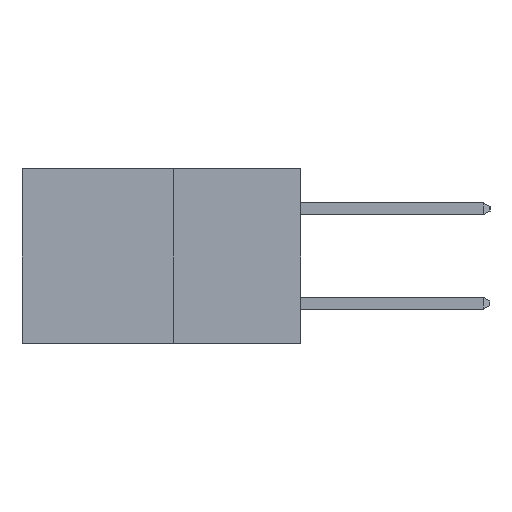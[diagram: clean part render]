
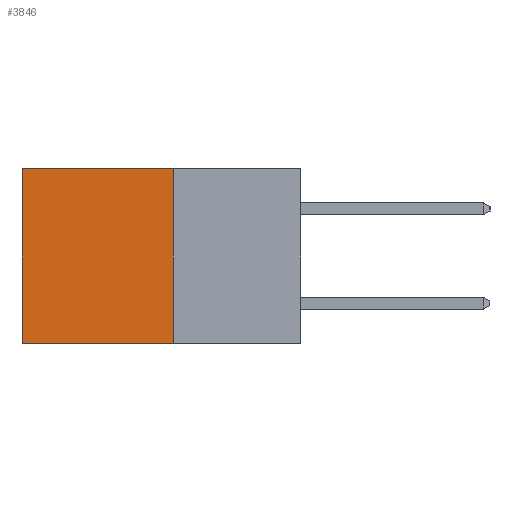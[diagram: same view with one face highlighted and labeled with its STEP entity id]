
A CAD part, left-side view. The second image highlights one B-rep face of the part: STEP entity #3846.
In plain terms, the highlighted planar face has unit normal (-1, 0, 0).
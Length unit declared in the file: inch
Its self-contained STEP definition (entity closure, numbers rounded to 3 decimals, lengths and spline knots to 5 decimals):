
#1355 = CARTESIAN_POINT ( 'NONE',  ( 0.277, 0.27, -0.37 ) ) ;
#2177 = LINE ( 'NONE', #3316, #24294 ) ;
#2244 = CARTESIAN_POINT ( 'NONE',  ( 0.277, 0.59, -0.37 ) ) ;
#3168 = EDGE_CURVE ( 'NONE', #17426, #20109, #24684, .T. ) ;
#3181 = DIRECTION ( 'NONE',  ( 0., 0., -1. ) ) ;
#3316 = CARTESIAN_POINT ( 'NONE',  ( 0.277, 0.59, -0.37 ) ) ;
#3846 = ADVANCED_FACE ( 'NONE', ( #8074 ), #18372, .F. ) ;
#5406 = ORIENTED_EDGE ( 'NONE', *, *, #13459, .F. ) ;
#6293 = EDGE_CURVE ( 'NONE', #20109, #27908, #2177, .T. ) ;
#6651 = EDGE_CURVE ( 'NONE', #17426, #11152, #9471, .T. ) ;
#7779 = VECTOR ( 'NONE', #15711, 39.37008 ) ;
#8074 = FACE_OUTER_BOUND ( 'NONE', #26539, .T. ) ;
#9471 = LINE ( 'NONE', #25321, #15317 ) ;
#11152 = VERTEX_POINT ( 'NONE', #25578 ) ;
#11865 = ORIENTED_EDGE ( 'NONE', *, *, #6651, .F. ) ;
#12144 = DIRECTION ( 'NONE',  ( 0., 0., -1. ) ) ;
#12700 = CARTESIAN_POINT ( 'NONE',  ( 0.277, 0.27, 0. ) ) ;
#12713 = ORIENTED_EDGE ( 'NONE', *, *, #3168, .T. ) ;
#12780 = CARTESIAN_POINT ( 'NONE',  ( 0.277, 0.59, 0. ) ) ;
#13048 = VECTOR ( 'NONE', #19036, 39.37008 ) ;
#13459 = EDGE_CURVE ( 'NONE', #11152, #27908, #19574, .T. ) ;
#14064 = ORIENTED_EDGE ( 'NONE', *, *, #6293, .T. ) ;
#15174 = AXIS2_PLACEMENT_3D ( 'NONE', #20018, #18273, #18241 ) ;
#15317 = VECTOR ( 'NONE', #12144, 39.37008 ) ;
#15711 = DIRECTION ( 'NONE',  ( 0., 1., 0. ) ) ;
#15801 = CARTESIAN_POINT ( 'NONE',  ( 0.277, 0.27, 0. ) ) ;
#17426 = VERTEX_POINT ( 'NONE', #12700 ) ;
#18241 = DIRECTION ( 'NONE',  ( 0., 0., -1. ) ) ;
#18273 = DIRECTION ( 'NONE',  ( 1., 0., 0. ) ) ;
#18372 = PLANE ( 'NONE',  #15174 ) ;
#19036 = DIRECTION ( 'NONE',  ( 0., 1., 0. ) ) ;
#19574 = LINE ( 'NONE', #1355, #13048 ) ;
#20018 = CARTESIAN_POINT ( 'NONE',  ( 0.277, 0.27, -0.37 ) ) ;
#20109 = VERTEX_POINT ( 'NONE', #12780 ) ;
#24294 = VECTOR ( 'NONE', #3181, 39.37008 ) ;
#24684 = LINE ( 'NONE', #15801, #7779 ) ;
#25321 = CARTESIAN_POINT ( 'NONE',  ( 0.277, 0.27, -0.37 ) ) ;
#25578 = CARTESIAN_POINT ( 'NONE',  ( 0.277, 0.27, -0.37 ) ) ;
#26539 = EDGE_LOOP ( 'NONE', ( #14064, #5406, #11865, #12713 ) ) ;
#27908 = VERTEX_POINT ( 'NONE', #2244 ) ;
